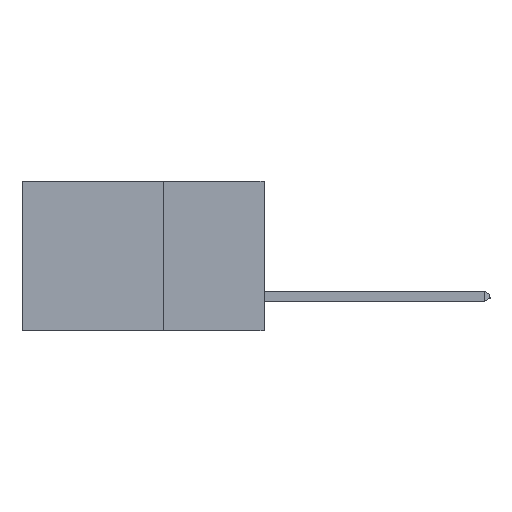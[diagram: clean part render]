
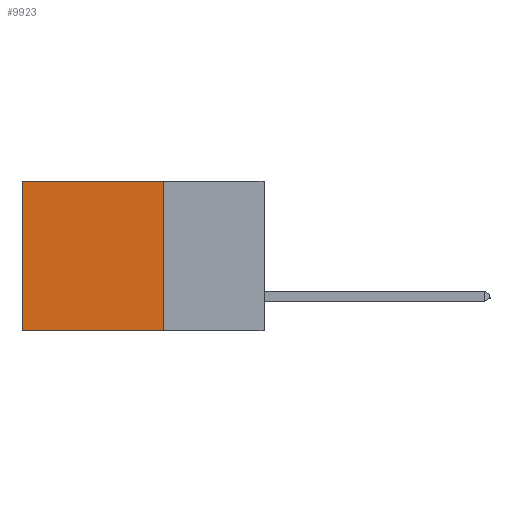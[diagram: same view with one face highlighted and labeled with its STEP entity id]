
A CAD part, left-side view. The second image highlights one B-rep face of the part: STEP entity #9923.
In plain terms, the highlighted planar face has unit normal (-1, 0, 0).
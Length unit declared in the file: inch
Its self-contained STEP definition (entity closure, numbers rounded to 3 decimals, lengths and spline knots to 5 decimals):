
#934 = CARTESIAN_POINT ( 'NONE',  ( 0.298, 0.25, 0. ) ) ;
#1429 = EDGE_CURVE ( 'NONE', #20042, #14362, #23928, .T. ) ;
#2165 = CARTESIAN_POINT ( 'NONE',  ( 0.298, 0.25, 0. ) ) ;
#2274 = VECTOR ( 'NONE', #20866, 39.37008 ) ;
#2692 = DIRECTION ( 'NONE',  ( 0., 0., -1. ) ) ;
#2716 = CARTESIAN_POINT ( 'NONE',  ( 0.298, 0.6, -0.37 ) ) ;
#2727 = ORIENTED_EDGE ( 'NONE', *, *, #1429, .F. ) ;
#7000 = ORIENTED_EDGE ( 'NONE', *, *, #21334, .T. ) ;
#8054 = ORIENTED_EDGE ( 'NONE', *, *, #17701, .T. ) ;
#8247 = LINE ( 'NONE', #934, #2274 ) ;
#8975 = DIRECTION ( 'NONE',  ( 0., 1., 0. ) ) ;
#9004 = VECTOR ( 'NONE', #19626, 39.37008 ) ;
#9923 = ADVANCED_FACE ( 'NONE', ( #26737 ), #26467, .F. ) ;
#13270 = ORIENTED_EDGE ( 'NONE', *, *, #15581, .F. ) ;
#13750 = CARTESIAN_POINT ( 'NONE',  ( 0.298, 0.25, 0. ) ) ;
#14362 = VERTEX_POINT ( 'NONE', #2716 ) ;
#15283 = VERTEX_POINT ( 'NONE', #18725 ) ;
#15581 = EDGE_CURVE ( 'NONE', #25276, #20042, #21102, .T. ) ;
#15880 = DIRECTION ( 'NONE',  ( 1., 0., 0. ) ) ;
#16241 = VECTOR ( 'NONE', #8975, 39.37008 ) ;
#16415 = DIRECTION ( 'NONE',  ( 0., 0., -1. ) ) ;
#17701 = EDGE_CURVE ( 'NONE', #25276, #15283, #8247, .T. ) ;
#18292 = EDGE_LOOP ( 'NONE', ( #7000, #2727, #13270, #8054 ) ) ;
#18474 = CARTESIAN_POINT ( 'NONE',  ( 0.298, 0.6, 0. ) ) ;
#18725 = CARTESIAN_POINT ( 'NONE',  ( 0.298, 0.6, 0. ) ) ;
#19626 = DIRECTION ( 'NONE',  ( 0., 0., -1. ) ) ;
#20042 = VERTEX_POINT ( 'NONE', #26808 ) ;
#20797 = VECTOR ( 'NONE', #16415, 39.37008 ) ;
#20866 = DIRECTION ( 'NONE',  ( 0., 1., 0. ) ) ;
#21102 = LINE ( 'NONE', #21854, #9004 ) ;
#21334 = EDGE_CURVE ( 'NONE', #15283, #14362, #26459, .T. ) ;
#21854 = CARTESIAN_POINT ( 'NONE',  ( 0.298, 0.25, 0. ) ) ;
#22691 = AXIS2_PLACEMENT_3D ( 'NONE', #13750, #15880, #2692 ) ;
#23291 = CARTESIAN_POINT ( 'NONE',  ( 0.298, 0.25, -0.37 ) ) ;
#23928 = LINE ( 'NONE', #23291, #16241 ) ;
#25276 = VERTEX_POINT ( 'NONE', #2165 ) ;
#26459 = LINE ( 'NONE', #18474, #20797 ) ;
#26467 = PLANE ( 'NONE',  #22691 ) ;
#26737 = FACE_OUTER_BOUND ( 'NONE', #18292, .T. ) ;
#26808 = CARTESIAN_POINT ( 'NONE',  ( 0.298, 0.25, -0.37 ) ) ;
